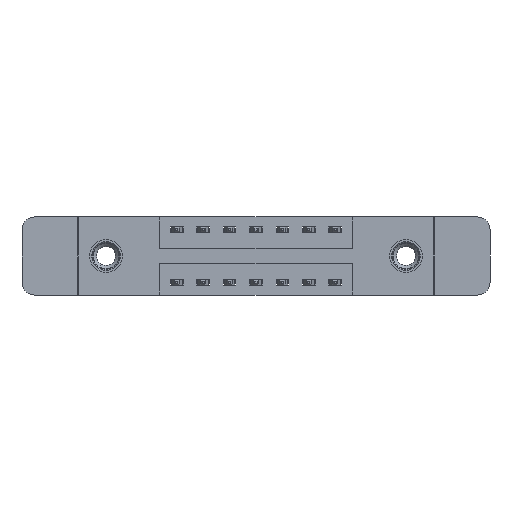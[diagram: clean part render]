
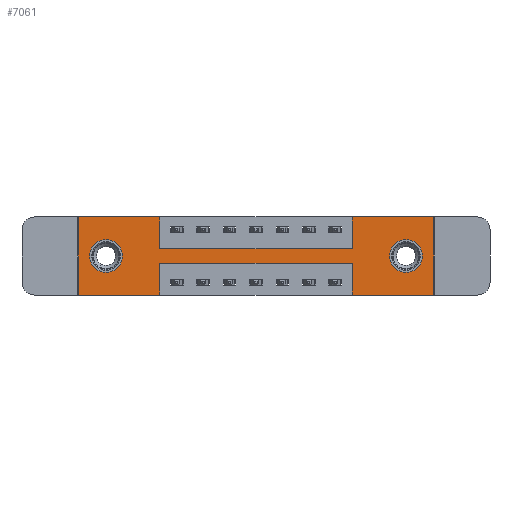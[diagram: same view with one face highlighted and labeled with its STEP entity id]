
A CAD part, front view. The second image highlights one B-rep face of the part: STEP entity #7061.
In plain terms, the highlighted planar face has unit normal (0, -1, 0).
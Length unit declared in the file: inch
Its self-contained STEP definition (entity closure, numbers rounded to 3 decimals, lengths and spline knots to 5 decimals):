
#100 = EDGE_CURVE ( 'NONE', #369, #7793, #13822, .T. ) ;
#157 = EDGE_CURVE ( 'NONE', #8649, #11855, #6805, .T. ) ;
#278 = LINE ( 'NONE', #9480, #11178 ) ;
#364 = AXIS2_PLACEMENT_3D ( 'NONE', #798, #4131, #4197 ) ;
#369 = VERTEX_POINT ( 'NONE', #9183 ) ;
#410 = LINE ( 'NONE', #7436, #7837 ) ;
#457 = ORIENTED_EDGE ( 'NONE', *, *, #13090, .F. ) ;
#557 = EDGE_LOOP ( 'NONE', ( #12059, #4702 ) ) ;
#752 = CARTESIAN_POINT ( 'NONE',  ( 1.2975, 0., -0.22 ) ) ;
#798 = CARTESIAN_POINT ( 'NONE',  ( 1.5525, 0., -0.185 ) ) ;
#840 = VECTOR ( 'NONE', #8167, 39.37008 ) ;
#1018 = DIRECTION ( 'NONE',  ( 0., 0., 1. ) ) ;
#1044 = VECTOR ( 'NONE', #5732, 39.37008 ) ;
#1122 = CARTESIAN_POINT ( 'NONE',  ( 1.685, 0., 0. ) ) ;
#1181 = VERTEX_POINT ( 'NONE', #12178 ) ;
#1191 = EDGE_CURVE ( 'NONE', #6077, #8649, #410, .T. ) ;
#1195 = EDGE_LOOP ( 'NONE', ( #13672, #457, #7191, #13993, #1601, #4213, #11809, #8688, #5082, #6245, #6845, #14827 ) ) ;
#1218 = CARTESIAN_POINT ( 'NONE',  ( 1.2975, 0., -0.37 ) ) ;
#1318 = EDGE_LOOP ( 'NONE', ( #12285, #11154 ) ) ;
#1400 = EDGE_CURVE ( 'NONE', #1181, #5844, #6671, .T. ) ;
#1514 = EDGE_CURVE ( 'NONE', #5844, #6915, #11561, .T. ) ;
#1601 = ORIENTED_EDGE ( 'NONE', *, *, #1982, .F. ) ;
#1890 = CARTESIAN_POINT ( 'NONE',  ( 0.3875, 0., 0. ) ) ;
#1982 = EDGE_CURVE ( 'NONE', #9218, #1181, #5957, .T. ) ;
#1995 = CARTESIAN_POINT ( 'NONE',  ( 0., 0., -0.37 ) ) ;
#2043 = CARTESIAN_POINT ( 'NONE',  ( 0.3875, 0., -0.37 ) ) ;
#2114 = VERTEX_POINT ( 'NONE', #13049 ) ;
#2219 = VERTEX_POINT ( 'NONE', #8893 ) ;
#2352 = DIRECTION ( 'NONE',  ( 0., 0., 1. ) ) ;
#2425 = EDGE_CURVE ( 'NONE', #12692, #6077, #278, .T. ) ;
#2473 = CARTESIAN_POINT ( 'NONE',  ( 0., 0., -0.37 ) ) ;
#3059 = EDGE_CURVE ( 'NONE', #8630, #12692, #9510, .T. ) ;
#3563 = CIRCLE ( 'NONE', #9605, 0.078 ) ;
#3609 = VECTOR ( 'NONE', #13452, 39.37008 ) ;
#3940 = LINE ( 'NONE', #5148, #11144 ) ;
#3995 = CIRCLE ( 'NONE', #364, 0.078 ) ;
#4131 = DIRECTION ( 'NONE',  ( 0., 1., 0. ) ) ;
#4197 = DIRECTION ( 'NONE',  ( 0., 0., -1. ) ) ;
#4213 = ORIENTED_EDGE ( 'NONE', *, *, #9560, .F. ) ;
#4341 = DIRECTION ( 'NONE',  ( 0., 1., 0. ) ) ;
#4531 = DIRECTION ( 'NONE',  ( 0., 1., 0. ) ) ;
#4660 = PLANE ( 'NONE',  #8648 ) ;
#4702 = ORIENTED_EDGE ( 'NONE', *, *, #10792, .T. ) ;
#4899 = DIRECTION ( 'NONE',  ( -1., 0., 0. ) ) ;
#5000 = EDGE_CURVE ( 'NONE', #11855, #2219, #6520, .T. ) ;
#5082 = ORIENTED_EDGE ( 'NONE', *, *, #157, .F. ) ;
#5148 = CARTESIAN_POINT ( 'NONE',  ( 0., 0., 0. ) ) ;
#5348 = CARTESIAN_POINT ( 'NONE',  ( 0.3875, 0., -0.22 ) ) ;
#5674 = CARTESIAN_POINT ( 'NONE',  ( 0.3875, 0., 0. ) ) ;
#5732 = DIRECTION ( 'NONE',  ( 0., 0., -1. ) ) ;
#5814 = EDGE_CURVE ( 'NONE', #8715, #2114, #3563, .T. ) ;
#5844 = VERTEX_POINT ( 'NONE', #10381 ) ;
#5895 = CARTESIAN_POINT ( 'NONE',  ( 1.5525, 0., -0.185 ) ) ;
#5957 = LINE ( 'NONE', #1122, #1044 ) ;
#6077 = VERTEX_POINT ( 'NONE', #14293 ) ;
#6245 = ORIENTED_EDGE ( 'NONE', *, *, #1191, .F. ) ;
#6408 = CARTESIAN_POINT ( 'NONE',  ( 0.1325, 0., -0.107 ) ) ;
#6520 = LINE ( 'NONE', #13387, #3609 ) ;
#6584 = DIRECTION ( 'NONE',  ( -1., 0., 0. ) ) ;
#6671 = LINE ( 'NONE', #1995, #12167 ) ;
#6805 = LINE ( 'NONE', #5674, #7815 ) ;
#6845 = ORIENTED_EDGE ( 'NONE', *, *, #2425, .F. ) ;
#6915 = VERTEX_POINT ( 'NONE', #752 ) ;
#7050 = CARTESIAN_POINT ( 'NONE',  ( 1.5525, 0., -0.263 ) ) ;
#7061 = ADVANCED_FACE ( 'NONE', ( #13635, #7919, #12513 ), #4660, .T. ) ;
#7156 = VERTEX_POINT ( 'NONE', #8366 ) ;
#7191 = ORIENTED_EDGE ( 'NONE', *, *, #1514, .F. ) ;
#7436 = CARTESIAN_POINT ( 'NONE',  ( 0., 0., 0. ) ) ;
#7793 = VERTEX_POINT ( 'NONE', #7050 ) ;
#7815 = VECTOR ( 'NONE', #11404, 39.37008 ) ;
#7837 = VECTOR ( 'NONE', #10972, 39.37008 ) ;
#7919 = FACE_BOUND ( 'NONE', #557, .T. ) ;
#7935 = DIRECTION ( 'NONE',  ( 0., 0., 1. ) ) ;
#7947 = CARTESIAN_POINT ( 'NONE',  ( 1.2975, 0., 0. ) ) ;
#8009 = EDGE_CURVE ( 'NONE', #2219, #7156, #12693, .T. ) ;
#8167 = DIRECTION ( 'NONE',  ( 0., 0., 1. ) ) ;
#8366 = CARTESIAN_POINT ( 'NONE',  ( 1.2975, 0., 0. ) ) ;
#8434 = DIRECTION ( 'NONE',  ( 0., 0., 1. ) ) ;
#8608 = CARTESIAN_POINT ( 'NONE',  ( 0., 0., -0.37 ) ) ;
#8630 = VERTEX_POINT ( 'NONE', #10930 ) ;
#8648 = AXIS2_PLACEMENT_3D ( 'NONE', #2473, #10476, #11603 ) ;
#8649 = VERTEX_POINT ( 'NONE', #1890 ) ;
#8688 = ORIENTED_EDGE ( 'NONE', *, *, #5000, .F. ) ;
#8715 = VERTEX_POINT ( 'NONE', #6408 ) ;
#8893 = CARTESIAN_POINT ( 'NONE',  ( 1.2975, 0., -0.15 ) ) ;
#9012 = CARTESIAN_POINT ( 'NONE',  ( 0., 0., -0.37 ) ) ;
#9016 = VECTOR ( 'NONE', #10109, 39.37008 ) ;
#9183 = CARTESIAN_POINT ( 'NONE',  ( 1.5525, 0., -0.107 ) ) ;
#9218 = VERTEX_POINT ( 'NONE', #14727 ) ;
#9339 = VECTOR ( 'NONE', #2352, 39.37008 ) ;
#9480 = CARTESIAN_POINT ( 'NONE',  ( 0., 0., 0. ) ) ;
#9510 = LINE ( 'NONE', #8608, #11400 ) ;
#9560 = EDGE_CURVE ( 'NONE', #7156, #9218, #3940, .T. ) ;
#9605 = AXIS2_PLACEMENT_3D ( 'NONE', #12564, #4341, #1018 ) ;
#10109 = DIRECTION ( 'NONE',  ( 0., 0., -1. ) ) ;
#10121 = CARTESIAN_POINT ( 'NONE',  ( 0.3875, 0., -0.22 ) ) ;
#10254 = CIRCLE ( 'NONE', #12189, 0.078 ) ;
#10340 = CARTESIAN_POINT ( 'NONE',  ( 0.1325, 0., -0.185 ) ) ;
#10381 = CARTESIAN_POINT ( 'NONE',  ( 1.2975, 0., -0.37 ) ) ;
#10457 = AXIS2_PLACEMENT_3D ( 'NONE', #5895, #4531, #11483 ) ;
#10476 = DIRECTION ( 'NONE',  ( 0., -1., 0. ) ) ;
#10792 = EDGE_CURVE ( 'NONE', #2114, #8715, #10254, .T. ) ;
#10930 = CARTESIAN_POINT ( 'NONE',  ( 0.3875, 0., -0.37 ) ) ;
#10972 = DIRECTION ( 'NONE',  ( 1., 0., 0. ) ) ;
#11144 = VECTOR ( 'NONE', #13360, 39.37008 ) ;
#11154 = ORIENTED_EDGE ( 'NONE', *, *, #13979, .T. ) ;
#11178 = VECTOR ( 'NONE', #8434, 39.37008 ) ;
#11400 = VECTOR ( 'NONE', #4899, 39.37008 ) ;
#11404 = DIRECTION ( 'NONE',  ( 0., 0., -1. ) ) ;
#11483 = DIRECTION ( 'NONE',  ( 0., 0., -1. ) ) ;
#11561 = LINE ( 'NONE', #1218, #840 ) ;
#11603 = DIRECTION ( 'NONE',  ( 0., 0., -1. ) ) ;
#11675 = VECTOR ( 'NONE', #12673, 39.37008 ) ;
#11809 = ORIENTED_EDGE ( 'NONE', *, *, #8009, .F. ) ;
#11855 = VERTEX_POINT ( 'NONE', #14628 ) ;
#12059 = ORIENTED_EDGE ( 'NONE', *, *, #5814, .T. ) ;
#12167 = VECTOR ( 'NONE', #6584, 39.37008 ) ;
#12178 = CARTESIAN_POINT ( 'NONE',  ( 1.685, 0., -0.37 ) ) ;
#12189 = AXIS2_PLACEMENT_3D ( 'NONE', #10340, #14785, #7935 ) ;
#12285 = ORIENTED_EDGE ( 'NONE', *, *, #100, .T. ) ;
#12513 = FACE_OUTER_BOUND ( 'NONE', #1195, .T. ) ;
#12520 = LINE ( 'NONE', #10121, #11675 ) ;
#12564 = CARTESIAN_POINT ( 'NONE',  ( 0.1325, 0., -0.185 ) ) ;
#12673 = DIRECTION ( 'NONE',  ( -1., 0., 0. ) ) ;
#12692 = VERTEX_POINT ( 'NONE', #9012 ) ;
#12693 = LINE ( 'NONE', #7947, #9339 ) ;
#13006 = EDGE_CURVE ( 'NONE', #13521, #8630, #14427, .T. ) ;
#13049 = CARTESIAN_POINT ( 'NONE',  ( 0.1325, 0., -0.263 ) ) ;
#13090 = EDGE_CURVE ( 'NONE', #6915, #13521, #12520, .T. ) ;
#13360 = DIRECTION ( 'NONE',  ( 1., 0., 0. ) ) ;
#13387 = CARTESIAN_POINT ( 'NONE',  ( 0.3875, 0., -0.15 ) ) ;
#13452 = DIRECTION ( 'NONE',  ( 1., 0., 0. ) ) ;
#13521 = VERTEX_POINT ( 'NONE', #5348 ) ;
#13635 = FACE_BOUND ( 'NONE', #1318, .T. ) ;
#13672 = ORIENTED_EDGE ( 'NONE', *, *, #13006, .F. ) ;
#13822 = CIRCLE ( 'NONE', #10457, 0.078 ) ;
#13979 = EDGE_CURVE ( 'NONE', #7793, #369, #3995, .T. ) ;
#13993 = ORIENTED_EDGE ( 'NONE', *, *, #1400, .F. ) ;
#14293 = CARTESIAN_POINT ( 'NONE',  ( 0., 0., 0. ) ) ;
#14427 = LINE ( 'NONE', #2043, #9016 ) ;
#14628 = CARTESIAN_POINT ( 'NONE',  ( 0.3875, 0., -0.15 ) ) ;
#14727 = CARTESIAN_POINT ( 'NONE',  ( 1.685, 0., 0. ) ) ;
#14785 = DIRECTION ( 'NONE',  ( 0., 1., 0. ) ) ;
#14827 = ORIENTED_EDGE ( 'NONE', *, *, #3059, .F. ) ;
